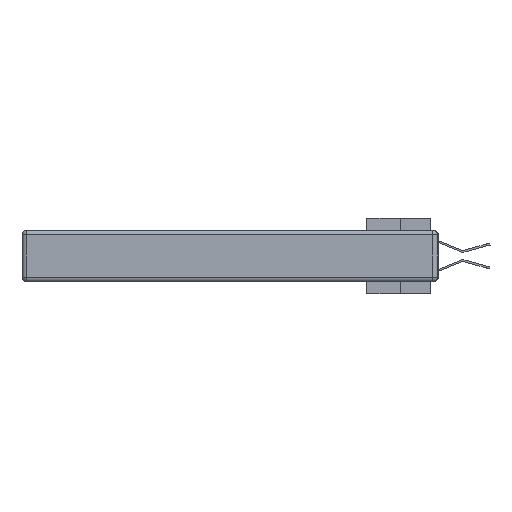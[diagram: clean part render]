
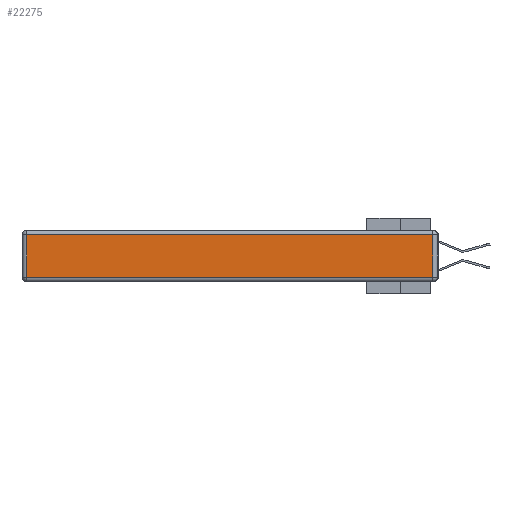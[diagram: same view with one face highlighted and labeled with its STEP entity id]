
A CAD part, left-side view. The second image highlights one B-rep face of the part: STEP entity #22275.
In plain terms, the highlighted planar face has unit normal (-1, 0, 0).
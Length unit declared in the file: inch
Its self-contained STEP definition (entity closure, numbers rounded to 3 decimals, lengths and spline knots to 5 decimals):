
#39 = VECTOR ( 'NONE', #11418, 39.37008 ) ;
#75 = LINE ( 'NONE', #14206, #39 ) ;
#1927 = EDGE_CURVE ( 'NONE', #32442, #28126, #17046, .T. ) ;
#2757 = DIRECTION ( 'NONE',  ( 0., 1., 0. ) ) ;
#3859 = VERTEX_POINT ( 'NONE', #5960 ) ;
#4445 = CARTESIAN_POINT ( 'NONE',  ( 0., 2.72, -0.343 ) ) ;
#5956 = FACE_OUTER_BOUND ( 'NONE', #24059, .T. ) ;
#5960 = CARTESIAN_POINT ( 'NONE',  ( 0., 2.72, -0.03 ) ) ;
#7844 = DIRECTION ( 'NONE',  ( 0., 0., 1. ) ) ;
#9761 = ORIENTED_EDGE ( 'NONE', *, *, #19384, .T. ) ;
#10552 = DIRECTION ( 'NONE',  ( 0., 0., 1. ) ) ;
#10937 = ORIENTED_EDGE ( 'NONE', *, *, #11037, .T. ) ;
#11037 = EDGE_CURVE ( 'NONE', #25373, #32442, #75, .T. ) ;
#11418 = DIRECTION ( 'NONE',  ( 0., -1., 0. ) ) ;
#11889 = DIRECTION ( 'NONE',  ( 0., 0., -1. ) ) ;
#14206 = CARTESIAN_POINT ( 'NONE',  ( 0., 0., -0.313 ) ) ;
#15457 = VECTOR ( 'NONE', #7844, 39.37008 ) ;
#17046 = LINE ( 'NONE', #18169, #15457 ) ;
#17480 = ORIENTED_EDGE ( 'NONE', *, *, #25895, .T. ) ;
#17594 = VECTOR ( 'NONE', #11889, 39.37008 ) ;
#18169 = CARTESIAN_POINT ( 'NONE',  ( 0., 0.03, -0.343 ) ) ;
#19384 = EDGE_CURVE ( 'NONE', #28126, #3859, #29778, .T. ) ;
#20164 = CARTESIAN_POINT ( 'NONE',  ( 0., 0., -0.343 ) ) ;
#20599 = DIRECTION ( 'NONE',  ( -1., 0., 0. ) ) ;
#20723 = VECTOR ( 'NONE', #2757, 39.37008 ) ;
#22054 = ORIENTED_EDGE ( 'NONE', *, *, #1927, .T. ) ;
#22275 = ADVANCED_FACE ( 'NONE', ( #5956 ), #23131, .T. ) ;
#22381 = CARTESIAN_POINT ( 'NONE',  ( 0., 2.72, -0.313 ) ) ;
#23131 = PLANE ( 'NONE',  #29657 ) ;
#24059 = EDGE_LOOP ( 'NONE', ( #10937, #22054, #9761, #17480 ) ) ;
#24291 = LINE ( 'NONE', #4445, #17594 ) ;
#25373 = VERTEX_POINT ( 'NONE', #22381 ) ;
#25620 = CARTESIAN_POINT ( 'NONE',  ( 0., 0.03, -0.03 ) ) ;
#25895 = EDGE_CURVE ( 'NONE', #3859, #25373, #24291, .T. ) ;
#28126 = VERTEX_POINT ( 'NONE', #25620 ) ;
#28235 = CARTESIAN_POINT ( 'NONE',  ( 0., 2.75, -0.03 ) ) ;
#28940 = CARTESIAN_POINT ( 'NONE',  ( 0., 0.03, -0.313 ) ) ;
#29657 = AXIS2_PLACEMENT_3D ( 'NONE', #20164, #20599, #10552 ) ;
#29778 = LINE ( 'NONE', #28235, #20723 ) ;
#32442 = VERTEX_POINT ( 'NONE', #28940 ) ;
